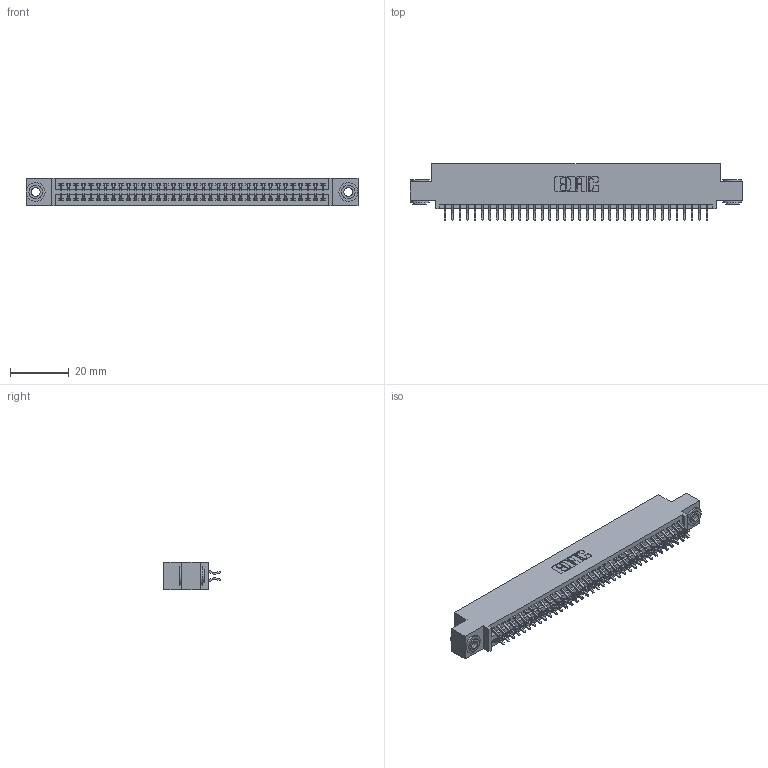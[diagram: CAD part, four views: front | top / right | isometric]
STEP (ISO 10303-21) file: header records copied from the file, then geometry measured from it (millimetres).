
FILE_DESCRIPTION (( 'STEP AP203' ), '1' );
FILE_NAME ('395-072-556-503.STEP', '2018-11-27T15:18:51', ( '' ), ( '' ), 'SwSTEP 2.0', 'SolidWorks 2016', '' );
FILE_SCHEMA (( 'CONFIG_CONTROL_DESIGN' ));
Length unit declared in the file: inch
Products named in the file (4): 345-250-002_345-250-002-102; 345-292-001_556 Tail; 395-072-556-503; 345 Part_0.110 Offset - 0.156 Dia-TH
Assembly tree (75 placements, depth 2):
  395-072-556-503
    345 Part_0.110 Offset - 0.156 Dia-TH
    345-292-001_556 Tail  x72
    345-250-002_345-250-002-102  x2
Bounding box: 112.65 x 19.24 x 9.4 mm (x, y, z)
Volume: 10830.3 mm3; surface area: 16127.5 mm2
Topology: 75 solids, 75 shells, 4200 faces, 12453 edges, 8202 vertices
Faces by surface type: plane 2758, cylinder 1434, cone 8
Entity records: 30056 total; most frequent: CARTESIAN_POINT 5035, ORIENTED_EDGE 4950, DIRECTION 4465, EDGE_CURVE 2475, VECTOR 2167, LINE 2167, VERTEX_POINT 1646, AXIS2_PLACEMENT_3D 1149
